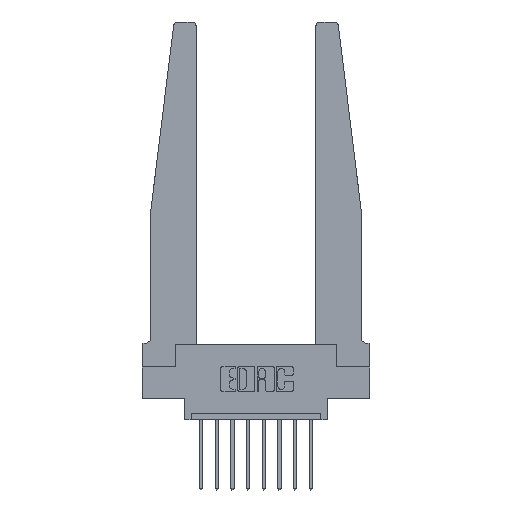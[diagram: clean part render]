
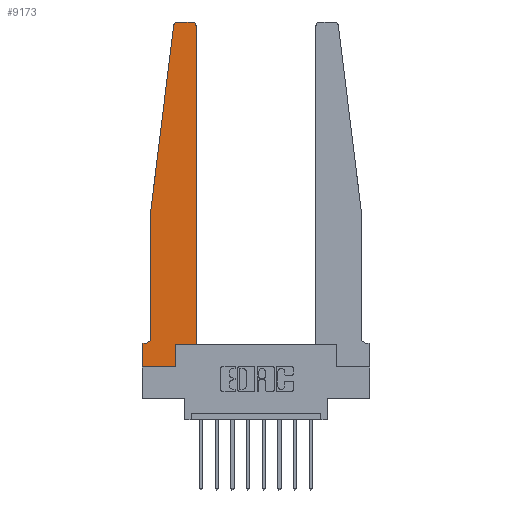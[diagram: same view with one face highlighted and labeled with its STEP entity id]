
A CAD part, top view. The second image highlights one B-rep face of the part: STEP entity #9173.
In plain terms, the highlighted planar face has unit normal (0, 0, 1).
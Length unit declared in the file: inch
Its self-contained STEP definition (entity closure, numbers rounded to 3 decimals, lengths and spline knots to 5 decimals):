
#31 = VECTOR ( 'NONE', #2587, 39.37008 ) ;
#129 = EDGE_CURVE ( 'NONE', #7623, #2370, #5160, .T. ) ;
#215 = CARTESIAN_POINT ( 'NONE',  ( 0., 0.1875, 0.37 ) ) ;
#260 = LINE ( 'NONE', #12952, #31 ) ;
#471 = CARTESIAN_POINT ( 'NONE',  ( 0.065, 0.1875, 0.37 ) ) ;
#504 = LINE ( 'NONE', #9992, #5498 ) ;
#667 = VECTOR ( 'NONE', #7603, 39.37008 ) ;
#1029 = ORIENTED_EDGE ( 'NONE', *, *, #14302, .T. ) ;
#1138 = EDGE_CURVE ( 'NONE', #7289, #5361, #5204, .T. ) ;
#1343 = EDGE_CURVE ( 'NONE', #3682, #10411, #13928, .T. ) ;
#1782 = CARTESIAN_POINT ( 'NONE',  ( 0.015, 0.1875, 0.37 ) ) ;
#1814 = ORIENTED_EDGE ( 'NONE', *, *, #4678, .T. ) ;
#2010 = DIRECTION ( 'NONE',  ( 1., 0., 0. ) ) ;
#2293 = DIRECTION ( 'NONE',  ( 0., 0., 1. ) ) ;
#2370 = VERTEX_POINT ( 'NONE', #4827 ) ;
#2581 = VECTOR ( 'NONE', #8555, 39.37008 ) ;
#2587 = DIRECTION ( 'NONE',  ( 0., -1., 0. ) ) ;
#2591 = CARTESIAN_POINT ( 'NONE',  ( 0.27653, 2.72, 0.37 ) ) ;
#2851 = CARTESIAN_POINT ( 'NONE',  ( 0., 0.1875, 0.37 ) ) ;
#3107 = CARTESIAN_POINT ( 'NONE',  ( 0.015, 0.2375, 0.37 ) ) ;
#3227 = EDGE_CURVE ( 'NONE', #10411, #7623, #9831, .T. ) ;
#3367 = EDGE_CURVE ( 'NONE', #2370, #6141, #14639, .T. ) ;
#3383 = ORIENTED_EDGE ( 'NONE', *, *, #8007, .T. ) ;
#3588 = CARTESIAN_POINT ( 'NONE',  ( 0.425, 0.18, 0.37 ) ) ;
#3682 = VERTEX_POINT ( 'NONE', #13847 ) ;
#3734 = ORIENTED_EDGE ( 'NONE', *, *, #4914, .T. ) ;
#3898 = VERTEX_POINT ( 'NONE', #1782 ) ;
#3928 = EDGE_CURVE ( 'NONE', #7310, #3682, #504, .T. ) ;
#4572 = LINE ( 'NONE', #11687, #8829 ) ;
#4670 = CARTESIAN_POINT ( 'NONE',  ( 0., 0., 0.37 ) ) ;
#4678 = EDGE_CURVE ( 'NONE', #3898, #7289, #8621, .T. ) ;
#4825 = DIRECTION ( 'NONE',  ( 1., 0., 0. ) ) ;
#4827 = CARTESIAN_POINT ( 'NONE',  ( 0.24675, 2.72367, 0.37 ) ) ;
#4902 = LINE ( 'NONE', #4670, #12736 ) ;
#4914 = EDGE_CURVE ( 'NONE', #5361, #6204, #4902, .T. ) ;
#5014 = DIRECTION ( 'NONE',  ( 1., 0., 0. ) ) ;
#5126 = AXIS2_PLACEMENT_3D ( 'NONE', #2851, #7478, #2010 ) ;
#5160 = CIRCLE ( 'NONE', #5394, 0.03 ) ;
#5204 = LINE ( 'NONE', #13613, #9358 ) ;
#5329 = CARTESIAN_POINT ( 'NONE',  ( 0.065, 0.2375, 0.37 ) ) ;
#5361 = VERTEX_POINT ( 'NONE', #13982 ) ;
#5394 = AXIS2_PLACEMENT_3D ( 'NONE', #2591, #11981, #5014 ) ;
#5498 = VECTOR ( 'NONE', #8729, 39.37008 ) ;
#6141 = VERTEX_POINT ( 'NONE', #12174 ) ;
#6204 = VERTEX_POINT ( 'NONE', #9877 ) ;
#6486 = ORIENTED_EDGE ( 'NONE', *, *, #3367, .T. ) ;
#6705 = VECTOR ( 'NONE', #13517, 39.37008 ) ;
#6798 = DIRECTION ( 'NONE',  ( 0., 1., 0. ) ) ;
#6849 = CARTESIAN_POINT ( 'NONE',  ( 0.395, 2.72, 0.37 ) ) ;
#6971 = ORIENTED_EDGE ( 'NONE', *, *, #13965, .T. ) ;
#7042 = CIRCLE ( 'NONE', #9431, 0.05 ) ;
#7164 = CARTESIAN_POINT ( 'NONE',  ( 0.27653, 2.75, 0.37 ) ) ;
#7253 = ORIENTED_EDGE ( 'NONE', *, *, #129, .T. ) ;
#7283 = DIRECTION ( 'NONE',  ( 1., 0., 0. ) ) ;
#7289 = VERTEX_POINT ( 'NONE', #215 ) ;
#7310 = VERTEX_POINT ( 'NONE', #3588 ) ;
#7453 = AXIS2_PLACEMENT_3D ( 'NONE', #6849, #2293, #13758 ) ;
#7478 = DIRECTION ( 'NONE',  ( 0., 0., 1. ) ) ;
#7566 = DIRECTION ( 'NONE',  ( 0., -1., 0. ) ) ;
#7603 = DIRECTION ( 'NONE',  ( -1., 0., 0. ) ) ;
#7623 = VERTEX_POINT ( 'NONE', #7164 ) ;
#8007 = EDGE_CURVE ( 'NONE', #6141, #9621, #260, .T. ) ;
#8263 = CARTESIAN_POINT ( 'NONE',  ( 0.425, 0.18, 0.37 ) ) ;
#8451 = EDGE_CURVE ( 'NONE', #9621, #3898, #7042, .T. ) ;
#8526 = VERTEX_POINT ( 'NONE', #11355 ) ;
#8555 = DIRECTION ( 'NONE',  ( -1., 0., 0. ) ) ;
#8621 = LINE ( 'NONE', #471, #2581 ) ;
#8729 = DIRECTION ( 'NONE',  ( 0., 1., 0. ) ) ;
#8829 = VECTOR ( 'NONE', #6798, 39.37008 ) ;
#8882 = FACE_OUTER_BOUND ( 'NONE', #11690, .T. ) ;
#8899 = CARTESIAN_POINT ( 'NONE',  ( 0.395, 2.75, 0.37 ) ) ;
#8922 = CARTESIAN_POINT ( 'NONE',  ( 0.065, 1.25, 0.37 ) ) ;
#9173 = ADVANCED_FACE ( 'NONE', ( #8882 ), #12373, .T. ) ;
#9358 = VECTOR ( 'NONE', #7566, 39.37008 ) ;
#9431 = AXIS2_PLACEMENT_3D ( 'NONE', #3107, #10273, #13745 ) ;
#9621 = VERTEX_POINT ( 'NONE', #5329 ) ;
#9831 = LINE ( 'NONE', #13163, #667 ) ;
#9877 = CARTESIAN_POINT ( 'NONE',  ( 0.2605, 0., 0.37 ) ) ;
#9992 = CARTESIAN_POINT ( 'NONE',  ( 0.425, 0.18, 0.37 ) ) ;
#10273 = DIRECTION ( 'NONE',  ( 0., 0., -1. ) ) ;
#10411 = VERTEX_POINT ( 'NONE', #8899 ) ;
#11355 = CARTESIAN_POINT ( 'NONE',  ( 0.2605, 0.18, 0.37 ) ) ;
#11687 = CARTESIAN_POINT ( 'NONE',  ( 0.2605, 0.18, 0.37 ) ) ;
#11690 = EDGE_LOOP ( 'NONE', ( #14372, #7253, #6486, #3383, #13402, #1814, #14674, #3734, #1029, #6971, #12702, #14454 ) ) ;
#11729 = VECTOR ( 'NONE', #7283, 39.37008 ) ;
#11981 = DIRECTION ( 'NONE',  ( 0., 0., 1. ) ) ;
#12174 = CARTESIAN_POINT ( 'NONE',  ( 0.065, 1.25, 0.37 ) ) ;
#12373 = PLANE ( 'NONE',  #5126 ) ;
#12702 = ORIENTED_EDGE ( 'NONE', *, *, #3928, .T. ) ;
#12736 = VECTOR ( 'NONE', #4825, 39.37008 ) ;
#12952 = CARTESIAN_POINT ( 'NONE',  ( 0.065, 1.25, 0.37 ) ) ;
#13163 = CARTESIAN_POINT ( 'NONE',  ( 0.25, 2.75, 0.37 ) ) ;
#13283 = LINE ( 'NONE', #8263, #11729 ) ;
#13402 = ORIENTED_EDGE ( 'NONE', *, *, #8451, .T. ) ;
#13517 = DIRECTION ( 'NONE',  ( -0.122, -0.992, 0. ) ) ;
#13613 = CARTESIAN_POINT ( 'NONE',  ( 0., 0., 0.37 ) ) ;
#13745 = DIRECTION ( 'NONE',  ( -1., 0., 0. ) ) ;
#13758 = DIRECTION ( 'NONE',  ( 1., 0., 0. ) ) ;
#13847 = CARTESIAN_POINT ( 'NONE',  ( 0.425, 2.72, 0.37 ) ) ;
#13928 = CIRCLE ( 'NONE', #7453, 0.03 ) ;
#13965 = EDGE_CURVE ( 'NONE', #8526, #7310, #13283, .T. ) ;
#13982 = CARTESIAN_POINT ( 'NONE',  ( 0., 0., 0.37 ) ) ;
#14302 = EDGE_CURVE ( 'NONE', #6204, #8526, #4572, .T. ) ;
#14372 = ORIENTED_EDGE ( 'NONE', *, *, #3227, .T. ) ;
#14454 = ORIENTED_EDGE ( 'NONE', *, *, #1343, .T. ) ;
#14639 = LINE ( 'NONE', #8922, #6705 ) ;
#14674 = ORIENTED_EDGE ( 'NONE', *, *, #1138, .T. ) ;
